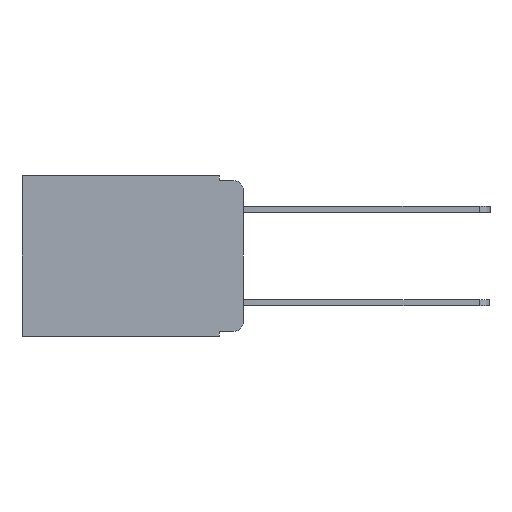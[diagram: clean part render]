
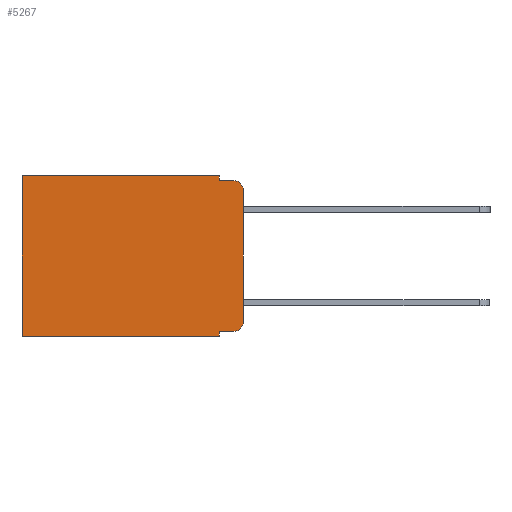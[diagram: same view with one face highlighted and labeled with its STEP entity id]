
A CAD part, left-side view. The second image highlights one B-rep face of the part: STEP entity #5267.
In plain terms, the highlighted planar face has unit normal (-1, 0, 0).
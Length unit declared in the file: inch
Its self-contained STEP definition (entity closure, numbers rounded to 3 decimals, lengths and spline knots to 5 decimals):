
#49 = CARTESIAN_POINT ( 'NONE',  ( 0.298, 0.051, -0.01 ) ) ;
#52 = DIRECTION ( 'NONE',  ( 0., -1., 0. ) ) ;
#134 = AXIS2_PLACEMENT_3D ( 'NONE', #10545, #10232, #5587 ) ;
#274 = VECTOR ( 'NONE', #6151, 39.37008 ) ;
#281 = EDGE_CURVE ( 'NONE', #7635, #7742, #8824, .T. ) ;
#308 = DIRECTION ( 'NONE',  ( 0., 1., 0. ) ) ;
#365 = DIRECTION ( 'NONE',  ( 0., 0., -1. ) ) ;
#391 = EDGE_LOOP ( 'NONE', ( #9994, #8362, #8152, #9617, #8448, #8507, #8542, #8193, #9088, #2902 ) ) ;
#544 = CARTESIAN_POINT ( 'NONE',  ( 0.298, 0.02, -0.03 ) ) ;
#656 = CARTESIAN_POINT ( 'NONE',  ( 0.298, 0.473, -0.343 ) ) ;
#931 = CARTESIAN_POINT ( 'NONE',  ( 0.298, 0., 0. ) ) ;
#1038 = CARTESIAN_POINT ( 'NONE',  ( 0.298, 0., -0.343 ) ) ;
#1105 = VERTEX_POINT ( 'NONE', #1181 ) ;
#1181 = CARTESIAN_POINT ( 'NONE',  ( 0.298, 0.051, -0.01 ) ) ;
#1256 = VECTOR ( 'NONE', #52, 39.37008 ) ;
#1304 = VECTOR ( 'NONE', #308, 39.37008 ) ;
#1350 = FACE_OUTER_BOUND ( 'NONE', #391, .T. ) ;
#1442 = CARTESIAN_POINT ( 'NONE',  ( 0.298, 0.051, 0. ) ) ;
#1462 = CARTESIAN_POINT ( 'NONE',  ( 0.298, 0.051, 0. ) ) ;
#1475 = DIRECTION ( 'NONE',  ( 0., 0., -1. ) ) ;
#1490 = CARTESIAN_POINT ( 'NONE',  ( 0.298, 0.02, -0.01 ) ) ;
#2016 = CARTESIAN_POINT ( 'NONE',  ( 0.298, 0., -0.03 ) ) ;
#2247 = CARTESIAN_POINT ( 'NONE',  ( 0.298, 0., 0. ) ) ;
#2281 = PLANE ( 'NONE',  #6952 ) ;
#2440 = CARTESIAN_POINT ( 'NONE',  ( 0.298, 0.02, -0.333 ) ) ;
#2624 = CARTESIAN_POINT ( 'NONE',  ( 0.298, 0.051, -0.333 ) ) ;
#2732 = EDGE_CURVE ( 'NONE', #5604, #3716, #9619, .T. ) ;
#2902 = ORIENTED_EDGE ( 'NONE', *, *, #7797, .T. ) ;
#3018 = EDGE_CURVE ( 'NONE', #5604, #7635, #3520, .T. ) ;
#3141 = VERTEX_POINT ( 'NONE', #1490 ) ;
#3173 = DIRECTION ( 'NONE',  ( 1., 0., 0. ) ) ;
#3195 = EDGE_CURVE ( 'NONE', #1105, #3141, #10008, .T. ) ;
#3299 = AXIS2_PLACEMENT_3D ( 'NONE', #544, #4133, #9672 ) ;
#3433 = VERTEX_POINT ( 'NONE', #5376 ) ;
#3520 = LINE ( 'NONE', #1462, #9633 ) ;
#3716 = VERTEX_POINT ( 'NONE', #2440 ) ;
#4133 = DIRECTION ( 'NONE',  ( -1., 0., 0. ) ) ;
#4555 = CARTESIAN_POINT ( 'NONE',  ( 0.298, 0.473, 0. ) ) ;
#4598 = CIRCLE ( 'NONE', #134, 0.02 ) ;
#4879 = VECTOR ( 'NONE', #6864, 39.37008 ) ;
#4895 = CARTESIAN_POINT ( 'NONE',  ( 0.298, 0.473, 0. ) ) ;
#5193 = DIRECTION ( 'NONE',  ( 0., 0., -1. ) ) ;
#5267 = ADVANCED_FACE ( 'NONE', ( #1350 ), #2281, .F. ) ;
#5376 = CARTESIAN_POINT ( 'NONE',  ( 0.298, 0., -0.313 ) ) ;
#5507 = VECTOR ( 'NONE', #9296, 39.37008 ) ;
#5587 = DIRECTION ( 'NONE',  ( 0., 0., -1. ) ) ;
#5604 = VERTEX_POINT ( 'NONE', #7936 ) ;
#6060 = CARTESIAN_POINT ( 'NONE',  ( 0.298, 0.051, -0.343 ) ) ;
#6151 = DIRECTION ( 'NONE',  ( 0., 0., -1. ) ) ;
#6413 = EDGE_CURVE ( 'NONE', #7862, #3433, #7160, .T. ) ;
#6831 = EDGE_CURVE ( 'NONE', #10739, #9288, #7716, .T. ) ;
#6864 = DIRECTION ( 'NONE',  ( 0., 1., 0. ) ) ;
#6900 = VECTOR ( 'NONE', #8118, 39.37008 ) ;
#6952 = AXIS2_PLACEMENT_3D ( 'NONE', #2247, #3173, #5193 ) ;
#7110 = EDGE_CURVE ( 'NONE', #9288, #7742, #7146, .T. ) ;
#7124 = EDGE_CURVE ( 'NONE', #7862, #3141, #7603, .T. ) ;
#7146 = LINE ( 'NONE', #4895, #6900 ) ;
#7160 = LINE ( 'NONE', #931, #274 ) ;
#7603 = CIRCLE ( 'NONE', #3299, 0.02 ) ;
#7635 = VERTEX_POINT ( 'NONE', #6060 ) ;
#7716 = LINE ( 'NONE', #7874, #1304 ) ;
#7742 = VERTEX_POINT ( 'NONE', #656 ) ;
#7797 = EDGE_CURVE ( 'NONE', #3716, #3433, #4598, .T. ) ;
#7862 = VERTEX_POINT ( 'NONE', #2016 ) ;
#7874 = CARTESIAN_POINT ( 'NONE',  ( 0.298, 0., 0. ) ) ;
#7936 = CARTESIAN_POINT ( 'NONE',  ( 0.298, 0.051, -0.333 ) ) ;
#8118 = DIRECTION ( 'NONE',  ( 0., 0., -1. ) ) ;
#8152 = ORIENTED_EDGE ( 'NONE', *, *, #3195, .F. ) ;
#8193 = ORIENTED_EDGE ( 'NONE', *, *, #3018, .F. ) ;
#8327 = LINE ( 'NONE', #9528, #10173 ) ;
#8362 = ORIENTED_EDGE ( 'NONE', *, *, #7124, .T. ) ;
#8448 = ORIENTED_EDGE ( 'NONE', *, *, #6831, .T. ) ;
#8507 = ORIENTED_EDGE ( 'NONE', *, *, #7110, .T. ) ;
#8542 = ORIENTED_EDGE ( 'NONE', *, *, #281, .F. ) ;
#8824 = LINE ( 'NONE', #1038, #4879 ) ;
#8995 = EDGE_CURVE ( 'NONE', #10739, #1105, #8327, .T. ) ;
#9088 = ORIENTED_EDGE ( 'NONE', *, *, #2732, .T. ) ;
#9288 = VERTEX_POINT ( 'NONE', #4555 ) ;
#9296 = DIRECTION ( 'NONE',  ( 0., -1., 0. ) ) ;
#9528 = CARTESIAN_POINT ( 'NONE',  ( 0.298, 0.051, 0. ) ) ;
#9617 = ORIENTED_EDGE ( 'NONE', *, *, #8995, .F. ) ;
#9619 = LINE ( 'NONE', #2624, #5507 ) ;
#9633 = VECTOR ( 'NONE', #1475, 39.37008 ) ;
#9672 = DIRECTION ( 'NONE',  ( 0., 0., -1. ) ) ;
#9994 = ORIENTED_EDGE ( 'NONE', *, *, #6413, .F. ) ;
#10008 = LINE ( 'NONE', #49, #1256 ) ;
#10173 = VECTOR ( 'NONE', #365, 39.37008 ) ;
#10232 = DIRECTION ( 'NONE',  ( -1., 0., 0. ) ) ;
#10545 = CARTESIAN_POINT ( 'NONE',  ( 0.298, 0.02, -0.313 ) ) ;
#10739 = VERTEX_POINT ( 'NONE', #1442 ) ;
